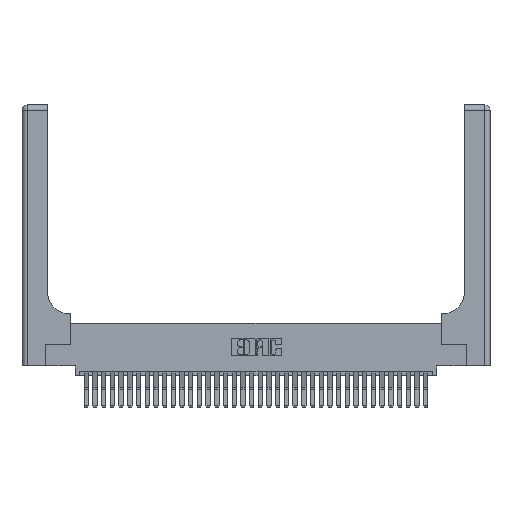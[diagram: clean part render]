
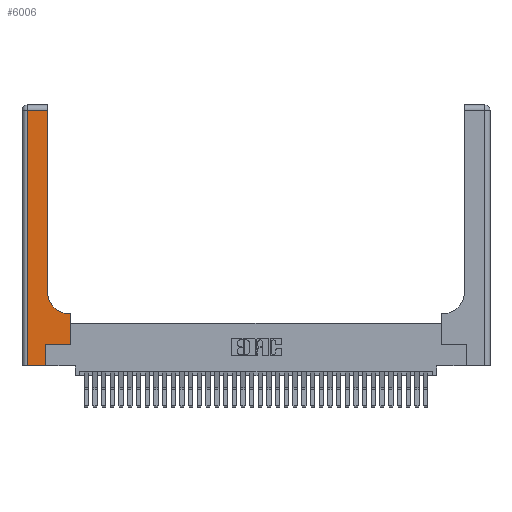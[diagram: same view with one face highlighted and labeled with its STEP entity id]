
A CAD part, top view. The second image highlights one B-rep face of the part: STEP entity #6006.
In plain terms, the highlighted planar face has unit normal (0, 0, 1).
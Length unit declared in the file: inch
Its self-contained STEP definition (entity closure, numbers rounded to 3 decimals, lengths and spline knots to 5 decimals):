
#274 = EDGE_CURVE ( 'NONE', #27826, #18394, #2776, .T. ) ;
#902 = LINE ( 'NONE', #12231, #33685 ) ;
#933 = DIRECTION ( 'NONE',  ( -1., 0., 0. ) ) ;
#1093 = DIRECTION ( 'NONE',  ( 0., 1., 0. ) ) ;
#2373 = VECTOR ( 'NONE', #25651, 39.37008 ) ;
#2559 = CARTESIAN_POINT ( 'NONE',  ( 0.269, 0., 0.37 ) ) ;
#2776 = CIRCLE ( 'NONE', #8986, 0.25 ) ;
#3020 = DIRECTION ( 'NONE',  ( 0., -1., 0. ) ) ;
#3839 = ORIENTED_EDGE ( 'NONE', *, *, #36491, .T. ) ;
#4016 = CARTESIAN_POINT ( 'NONE',  ( 0., 2.94, 0.37 ) ) ;
#4542 = ORIENTED_EDGE ( 'NONE', *, *, #7185, .T. ) ;
#4725 = CARTESIAN_POINT ( 'NONE',  ( 0.2915, 0.6, 0.37 ) ) ;
#4940 = CARTESIAN_POINT ( 'NONE',  ( 0.269, 0., 0.37 ) ) ;
#5059 = ORIENTED_EDGE ( 'NONE', *, *, #16937, .T. ) ;
#5201 = DIRECTION ( 'NONE',  ( 0., 1., 0. ) ) ;
#5664 = CARTESIAN_POINT ( 'NONE',  ( 0., 0., 0.37 ) ) ;
#5790 = CARTESIAN_POINT ( 'NONE',  ( 0.5585, 0.6, 0.37 ) ) ;
#6006 = ADVANCED_FACE ( 'NONE', ( #32239 ), #18157, .F. ) ;
#6627 = CARTESIAN_POINT ( 'NONE',  ( 0.269, 0.25, 0.37 ) ) ;
#7185 = EDGE_CURVE ( 'NONE', #18394, #7577, #11223, .T. ) ;
#7577 = VERTEX_POINT ( 'NONE', #16312 ) ;
#7869 = DIRECTION ( 'NONE',  ( 0., 0., -1. ) ) ;
#8084 = VECTOR ( 'NONE', #5201, 39.37008 ) ;
#8986 = AXIS2_PLACEMENT_3D ( 'NONE', #24987, #7869, #10997 ) ;
#9467 = DIRECTION ( 'NONE',  ( 0., 0., -1. ) ) ;
#10048 = CARTESIAN_POINT ( 'NONE',  ( 0.06, 2.94, 0.37 ) ) ;
#10417 = CARTESIAN_POINT ( 'NONE',  ( 0.5415, 0.6, 0.37 ) ) ;
#10997 = DIRECTION ( 'NONE',  ( 1., 0., 0. ) ) ;
#10998 = VERTEX_POINT ( 'NONE', #30177 ) ;
#11135 = AXIS2_PLACEMENT_3D ( 'NONE', #15458, #9467, #33099 ) ;
#11223 = LINE ( 'NONE', #32529, #18721 ) ;
#12231 = CARTESIAN_POINT ( 'NONE',  ( 0.5585, 0.25, 0.37 ) ) ;
#12424 = EDGE_CURVE ( 'NONE', #34467, #27826, #14173, .T. ) ;
#14173 = LINE ( 'NONE', #4725, #32390 ) ;
#14248 = VERTEX_POINT ( 'NONE', #6627 ) ;
#14278 = ORIENTED_EDGE ( 'NONE', *, *, #36869, .T. ) ;
#14472 = EDGE_CURVE ( 'NONE', #19085, #34467, #902, .T. ) ;
#14709 = LINE ( 'NONE', #4940, #8084 ) ;
#14866 = LINE ( 'NONE', #5664, #2373 ) ;
#15458 = CARTESIAN_POINT ( 'NONE',  ( 0., 3., 0.37 ) ) ;
#16312 = CARTESIAN_POINT ( 'NONE',  ( 0.2915, 2.94, 0.37 ) ) ;
#16937 = EDGE_CURVE ( 'NONE', #14248, #19085, #17300, .T. ) ;
#17056 = VERTEX_POINT ( 'NONE', #10048 ) ;
#17300 = LINE ( 'NONE', #22293, #23131 ) ;
#18157 = PLANE ( 'NONE',  #11135 ) ;
#18394 = VERTEX_POINT ( 'NONE', #24094 ) ;
#18721 = VECTOR ( 'NONE', #1093, 39.37008 ) ;
#19013 = CARTESIAN_POINT ( 'NONE',  ( 0.5585, 0.25, 0.37 ) ) ;
#19085 = VERTEX_POINT ( 'NONE', #19013 ) ;
#20951 = ORIENTED_EDGE ( 'NONE', *, *, #26774, .T. ) ;
#21863 = EDGE_CURVE ( 'NONE', #35660, #14248, #14709, .T. ) ;
#22293 = CARTESIAN_POINT ( 'NONE',  ( 0.269, 0.25, 0.37 ) ) ;
#23131 = VECTOR ( 'NONE', #27815, 39.37008 ) ;
#23462 = LINE ( 'NONE', #36840, #27544 ) ;
#24094 = CARTESIAN_POINT ( 'NONE',  ( 0.2915, 0.85, 0.37 ) ) ;
#24396 = VECTOR ( 'NONE', #933, 39.37008 ) ;
#24987 = CARTESIAN_POINT ( 'NONE',  ( 0.5415, 0.85, 0.37 ) ) ;
#25276 = EDGE_LOOP ( 'NONE', ( #4542, #3839, #14278, #20951, #36658, #5059, #26694, #34844, #33194 ) ) ;
#25651 = DIRECTION ( 'NONE',  ( 1., 0., 0. ) ) ;
#26694 = ORIENTED_EDGE ( 'NONE', *, *, #14472, .T. ) ;
#26774 = EDGE_CURVE ( 'NONE', #10998, #35660, #14866, .T. ) ;
#27544 = VECTOR ( 'NONE', #3020, 39.37008 ) ;
#27815 = DIRECTION ( 'NONE',  ( 1., 0., 0. ) ) ;
#27826 = VERTEX_POINT ( 'NONE', #10417 ) ;
#30176 = DIRECTION ( 'NONE',  ( -1., 0., 0. ) ) ;
#30177 = CARTESIAN_POINT ( 'NONE',  ( 0.06, 0., 0.37 ) ) ;
#30730 = LINE ( 'NONE', #4016, #24396 ) ;
#32239 = FACE_OUTER_BOUND ( 'NONE', #25276, .T. ) ;
#32390 = VECTOR ( 'NONE', #30176, 39.37008 ) ;
#32529 = CARTESIAN_POINT ( 'NONE',  ( 0.2915, 3., 0.37 ) ) ;
#33099 = DIRECTION ( 'NONE',  ( -1., 0., 0. ) ) ;
#33194 = ORIENTED_EDGE ( 'NONE', *, *, #274, .T. ) ;
#33685 = VECTOR ( 'NONE', #35261, 39.37008 ) ;
#34467 = VERTEX_POINT ( 'NONE', #5790 ) ;
#34844 = ORIENTED_EDGE ( 'NONE', *, *, #12424, .T. ) ;
#35261 = DIRECTION ( 'NONE',  ( 0., 1., 0. ) ) ;
#35660 = VERTEX_POINT ( 'NONE', #2559 ) ;
#36491 = EDGE_CURVE ( 'NONE', #7577, #17056, #30730, .T. ) ;
#36658 = ORIENTED_EDGE ( 'NONE', *, *, #21863, .T. ) ;
#36840 = CARTESIAN_POINT ( 'NONE',  ( 0.06, 3., 0.37 ) ) ;
#36869 = EDGE_CURVE ( 'NONE', #17056, #10998, #23462, .T. ) ;
